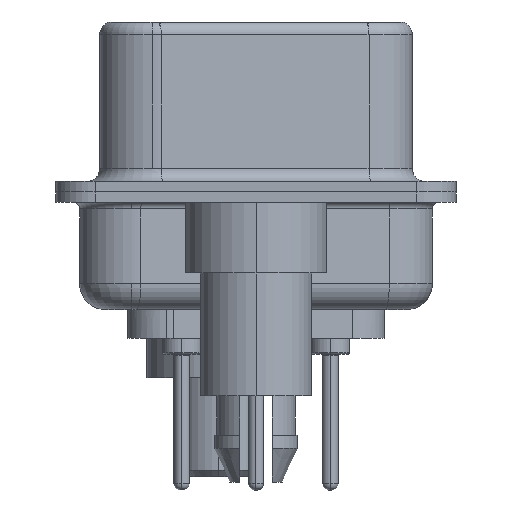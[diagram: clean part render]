
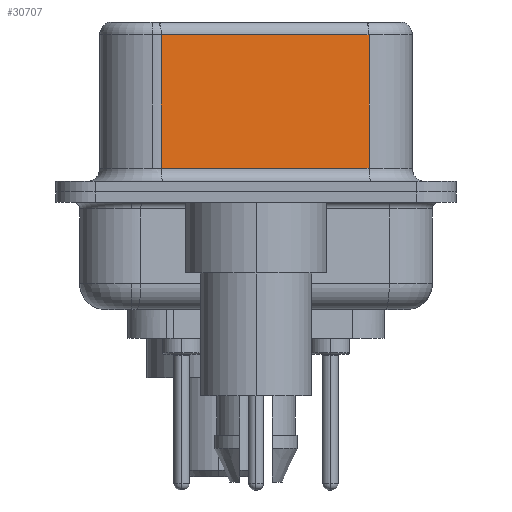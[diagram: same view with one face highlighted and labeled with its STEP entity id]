
A CAD part, left-side view. The second image highlights one B-rep face of the part: STEP entity #30707.
In plain terms, the highlighted planar face has unit normal (-0.985, -0.174, 0).
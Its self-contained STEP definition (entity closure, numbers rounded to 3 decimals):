
#133 = CARTESIAN_POINT ( 'NONE',  ( 5.132, -4.322, 6.02 ) ) ;
#151 = DIRECTION ( 'NONE',  ( -0.174, 0.985, 0. ) ) ;
#2218 = EDGE_CURVE ( 'NONE', #31835, #16542, #28007, .T. ) ;
#2392 = DIRECTION ( 'NONE',  ( 0.985, 0.174, 0. ) ) ;
#4113 = EDGE_LOOP ( 'NONE', ( #17381, #26019, #4310, #32344 ) ) ;
#4310 = ORIENTED_EDGE ( 'NONE', *, *, #2218, .T. ) ;
#4509 = CARTESIAN_POINT ( 'NONE',  ( 5.132, -4.322, 0.9 ) ) ;
#4879 = LINE ( 'NONE', #133, #14817 ) ;
#5475 = VECTOR ( 'NONE', #14777, 1000. ) ;
#5833 = EDGE_CURVE ( 'NONE', #15179, #31835, #4879, .T. ) ;
#7494 = DIRECTION ( 'NONE',  ( 0., 0., -1. ) ) ;
#10040 = CARTESIAN_POINT ( 'NONE',  ( 3.73, 3.628, 6.52 ) ) ;
#10519 = CARTESIAN_POINT ( 'NONE',  ( 5.132, -4.322, 6.52 ) ) ;
#10804 = EDGE_CURVE ( 'NONE', #16542, #30448, #33394, .T. ) ;
#10865 = CARTESIAN_POINT ( 'NONE',  ( 5.132, -4.322, 6.02 ) ) ;
#11235 = AXIS2_PLACEMENT_3D ( 'NONE', #10519, #2392, #151 ) ;
#12784 = CARTESIAN_POINT ( 'NONE',  ( 5.132, -4.322, 6.52 ) ) ;
#13003 = DIRECTION ( 'NONE',  ( 0., 0., -1. ) ) ;
#14757 = CARTESIAN_POINT ( 'NONE',  ( 3.73, 3.628, 0.9 ) ) ;
#14777 = DIRECTION ( 'NONE',  ( 0.174, -0.985, 0. ) ) ;
#14817 = VECTOR ( 'NONE', #29688, 1000. ) ;
#15179 = VERTEX_POINT ( 'NONE', #10865 ) ;
#16542 = VERTEX_POINT ( 'NONE', #14757 ) ;
#17381 = ORIENTED_EDGE ( 'NONE', *, *, #22672, .F. ) ;
#19213 = VECTOR ( 'NONE', #7494, 1000. ) ;
#20213 = CARTESIAN_POINT ( 'NONE',  ( 5.132, -4.322, 0.9 ) ) ;
#21688 = FACE_OUTER_BOUND ( 'NONE', #4113, .T. ) ;
#22672 = EDGE_CURVE ( 'NONE', #15179, #30448, #28908, .T. ) ;
#26019 = ORIENTED_EDGE ( 'NONE', *, *, #5833, .T. ) ;
#26436 = PLANE ( 'NONE',  #11235 ) ;
#28007 = LINE ( 'NONE', #10040, #19213 ) ;
#28471 = VECTOR ( 'NONE', #13003, 1000. ) ;
#28908 = LINE ( 'NONE', #12784, #28471 ) ;
#28942 = CARTESIAN_POINT ( 'NONE',  ( 3.73, 3.628, 6.02 ) ) ;
#29688 = DIRECTION ( 'NONE',  ( -0.174, 0.985, 0. ) ) ;
#30448 = VERTEX_POINT ( 'NONE', #4509 ) ;
#30707 = ADVANCED_FACE ( 'NONE', ( #21688 ), #26436, .F. ) ;
#31835 = VERTEX_POINT ( 'NONE', #28942 ) ;
#32344 = ORIENTED_EDGE ( 'NONE', *, *, #10804, .T. ) ;
#33394 = LINE ( 'NONE', #20213, #5475 ) ;
